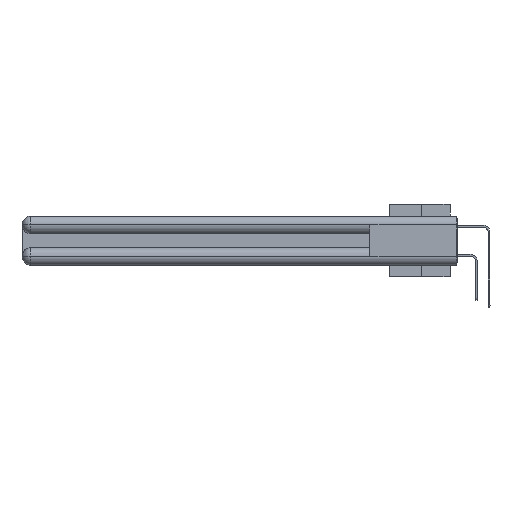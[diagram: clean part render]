
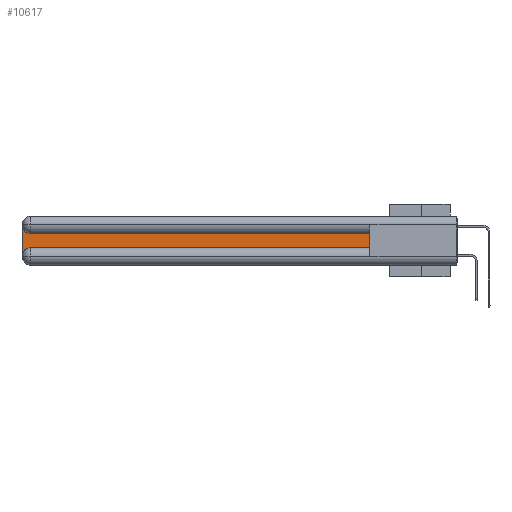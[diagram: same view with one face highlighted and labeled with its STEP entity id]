
A CAD part, left-side view. The second image highlights one B-rep face of the part: STEP entity #10617.
In plain terms, the highlighted planar face has unit normal (-1, 0, 0).
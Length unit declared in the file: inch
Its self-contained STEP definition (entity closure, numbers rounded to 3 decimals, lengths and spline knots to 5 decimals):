
#245 = VERTEX_POINT ( 'NONE', #23471 ) ;
#690 = AXIS2_PLACEMENT_3D ( 'NONE', #25906, #26222, #10334 ) ;
#994 = VERTEX_POINT ( 'NONE', #30579 ) ;
#1475 = LINE ( 'NONE', #22018, #24409 ) ;
#2451 = EDGE_CURVE ( 'NONE', #994, #245, #1475, .T. ) ;
#2705 = ORIENTED_EDGE ( 'NONE', *, *, #31397, .T. ) ;
#3254 = CARTESIAN_POINT ( 'NONE',  ( 0.075, 0.6, -0.1225 ) ) ;
#4860 = FACE_OUTER_BOUND ( 'NONE', #25623, .T. ) ;
#5849 = ORIENTED_EDGE ( 'NONE', *, *, #23825, .T. ) ;
#6141 = ORIENTED_EDGE ( 'NONE', *, *, #2451, .T. ) ;
#7351 = EDGE_CURVE ( 'NONE', #20453, #27494, #28477, .T. ) ;
#7992 = LINE ( 'NONE', #25546, #25003 ) ;
#9777 = VECTOR ( 'NONE', #22236, 39.37008 ) ;
#10206 = CARTESIAN_POINT ( 'NONE',  ( 0.075, 0.6, -0.2175 ) ) ;
#10334 = DIRECTION ( 'NONE',  ( 0., 0., -1. ) ) ;
#10410 = CARTESIAN_POINT ( 'NONE',  ( 0.075, 2.94, -0.0625 ) ) ;
#10617 = ADVANCED_FACE ( 'NONE', ( #4860 ), #25247, .F. ) ;
#13694 = CARTESIAN_POINT ( 'NONE',  ( 0.075, 3., -0.0625 ) ) ;
#14660 = DIRECTION ( 'NONE',  ( 0., -1., 0. ) ) ;
#15015 = EDGE_CURVE ( 'NONE', #245, #23965, #30441, .T. ) ;
#15904 = CARTESIAN_POINT ( 'NONE',  ( 0.075, 3., -0.2175 ) ) ;
#18157 = DIRECTION ( 'NONE',  ( 0., 1., 0. ) ) ;
#20453 = VERTEX_POINT ( 'NONE', #13694 ) ;
#20894 = CIRCLE ( 'NONE', #31061, 0.06 ) ;
#20902 = ORIENTED_EDGE ( 'NONE', *, *, #25856, .T. ) ;
#22018 = CARTESIAN_POINT ( 'NONE',  ( 0.075, 0.6, -0.2175 ) ) ;
#22236 = DIRECTION ( 'NONE',  ( 0., 0., 1. ) ) ;
#22563 = CARTESIAN_POINT ( 'NONE',  ( 0.075, 3., -0.1225 ) ) ;
#22627 = DIRECTION ( 'NONE',  ( 0., 0., -1. ) ) ;
#22670 = DIRECTION ( 'NONE',  ( 0., 0., -1. ) ) ;
#23471 = CARTESIAN_POINT ( 'NONE',  ( 0.075, 0.6, -0.2175 ) ) ;
#23678 = CARTESIAN_POINT ( 'NONE',  ( 0.075, 3., -0.2775 ) ) ;
#23825 = EDGE_CURVE ( 'NONE', #29855, #20453, #20894, .T. ) ;
#23965 = VERTEX_POINT ( 'NONE', #3254 ) ;
#24409 = VECTOR ( 'NONE', #14660, 39.37008 ) ;
#24597 = AXIS2_PLACEMENT_3D ( 'NONE', #22563, #30239, #32926 ) ;
#25003 = VECTOR ( 'NONE', #18157, 39.37008 ) ;
#25164 = ORIENTED_EDGE ( 'NONE', *, *, #15015, .T. ) ;
#25247 = PLANE ( 'NONE',  #24597 ) ;
#25309 = ORIENTED_EDGE ( 'NONE', *, *, #7351, .T. ) ;
#25546 = CARTESIAN_POINT ( 'NONE',  ( 0.075, 0.6, -0.1225 ) ) ;
#25591 = VECTOR ( 'NONE', #22670, 39.37008 ) ;
#25623 = EDGE_LOOP ( 'NONE', ( #2705, #5849, #25309, #20902, #6141, #25164 ) ) ;
#25856 = EDGE_CURVE ( 'NONE', #27494, #994, #32707, .T. ) ;
#25906 = CARTESIAN_POINT ( 'NONE',  ( 0.075, 2.94, -0.2775 ) ) ;
#26222 = DIRECTION ( 'NONE',  ( 1., 0., 0. ) ) ;
#27494 = VERTEX_POINT ( 'NONE', #23678 ) ;
#27973 = DIRECTION ( 'NONE',  ( 1., 0., 0. ) ) ;
#28477 = LINE ( 'NONE', #15904, #25591 ) ;
#29855 = VERTEX_POINT ( 'NONE', #31487 ) ;
#30239 = DIRECTION ( 'NONE',  ( 1., 0., 0. ) ) ;
#30441 = LINE ( 'NONE', #10206, #9777 ) ;
#30579 = CARTESIAN_POINT ( 'NONE',  ( 0.075, 2.94, -0.2175 ) ) ;
#31061 = AXIS2_PLACEMENT_3D ( 'NONE', #10410, #27973, #22627 ) ;
#31397 = EDGE_CURVE ( 'NONE', #23965, #29855, #7992, .T. ) ;
#31487 = CARTESIAN_POINT ( 'NONE',  ( 0.075, 2.94, -0.1225 ) ) ;
#32707 = CIRCLE ( 'NONE', #690, 0.06 ) ;
#32926 = DIRECTION ( 'NONE',  ( 0., 0., -1. ) ) ;
